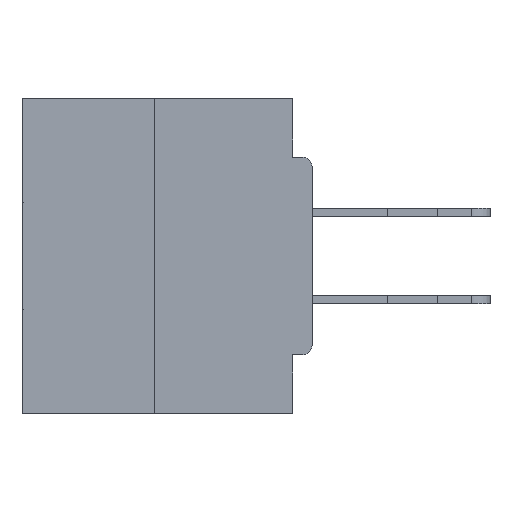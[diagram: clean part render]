
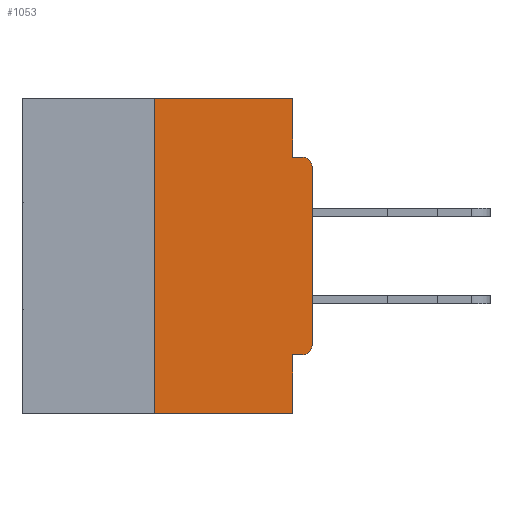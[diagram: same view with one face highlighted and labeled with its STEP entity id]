
A CAD part, left-side view. The second image highlights one B-rep face of the part: STEP entity #1053.
In plain terms, the highlighted planar face has unit normal (-1, 0, 0).
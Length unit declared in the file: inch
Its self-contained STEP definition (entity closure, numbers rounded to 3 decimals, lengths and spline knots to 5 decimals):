
#643 = VECTOR ( 'NONE', #5961, 39.37008 ) ;
#1053 = ADVANCED_FACE ( 'NONE', ( #13274 ), #39040, .F. ) ;
#1086 = EDGE_CURVE ( 'NONE', #33761, #31400, #2403, .T. ) ;
#2324 = CARTESIAN_POINT ( 'NONE',  ( 0., 0.46, 0. ) ) ;
#2388 = ORIENTED_EDGE ( 'NONE', *, *, #25637, .F. ) ;
#2403 = CIRCLE ( 'NONE', #8850, 0.015 ) ;
#2561 = DIRECTION ( 'NONE',  ( 0., 1., 0. ) ) ;
#2689 = CARTESIAN_POINT ( 'NONE',  ( 0., 0., -0.4065 ) ) ;
#2743 = EDGE_CURVE ( 'NONE', #36483, #14651, #9310, .T. ) ;
#2837 = DIRECTION ( 'NONE',  ( 0., 0., -1. ) ) ;
#3493 = LINE ( 'NONE', #24040, #643 ) ;
#4959 = VECTOR ( 'NONE', #20581, 39.37008 ) ;
#5961 = DIRECTION ( 'NONE',  ( 0., -1., 0. ) ) ;
#6221 = CARTESIAN_POINT ( 'NONE',  ( 0., 0.25, 0. ) ) ;
#6456 = LINE ( 'NONE', #2689, #19626 ) ;
#7245 = ORIENTED_EDGE ( 'NONE', *, *, #2743, .F. ) ;
#7557 = CARTESIAN_POINT ( 'NONE',  ( 0., 0.031, 0. ) ) ;
#7920 = CARTESIAN_POINT ( 'NONE',  ( 0., 0.46, -0.5 ) ) ;
#8850 = AXIS2_PLACEMENT_3D ( 'NONE', #31286, #16060, #36761 ) ;
#9133 = LINE ( 'NONE', #10523, #34714 ) ;
#9310 = LINE ( 'NONE', #14840, #13124 ) ;
#9994 = ORIENTED_EDGE ( 'NONE', *, *, #1086, .T. ) ;
#10086 = CARTESIAN_POINT ( 'NONE',  ( 0., 0., -0.3915 ) ) ;
#10115 = CARTESIAN_POINT ( 'NONE',  ( 0., 0.031, 0. ) ) ;
#10317 = DIRECTION ( 'NONE',  ( 0., 0., -1. ) ) ;
#10523 = CARTESIAN_POINT ( 'NONE',  ( 0., 0., 0. ) ) ;
#10832 = LINE ( 'NONE', #7920, #22151 ) ;
#11021 = VERTEX_POINT ( 'NONE', #20688 ) ;
#11458 = VERTEX_POINT ( 'NONE', #10115 ) ;
#11491 = LINE ( 'NONE', #6221, #30450 ) ;
#12255 = EDGE_LOOP ( 'NONE', ( #38855, #14845, #33498, #7245, #28476, #9994, #30283, #31205, #2388, #26505 ) ) ;
#13124 = VECTOR ( 'NONE', #21184, 39.37008 ) ;
#13274 = FACE_OUTER_BOUND ( 'NONE', #12255, .T. ) ;
#14538 = CARTESIAN_POINT ( 'NONE',  ( 0., 0.46, 0. ) ) ;
#14651 = VERTEX_POINT ( 'NONE', #38196 ) ;
#14840 = CARTESIAN_POINT ( 'NONE',  ( 0., 0.031, -0.5 ) ) ;
#14845 = ORIENTED_EDGE ( 'NONE', *, *, #35060, .F. ) ;
#14917 = DIRECTION ( 'NONE',  ( 1., 0., 0. ) ) ;
#15110 = DIRECTION ( 'NONE',  ( -1., 0., 0. ) ) ;
#15507 = EDGE_CURVE ( 'NONE', #11458, #36662, #22193, .T. ) ;
#15637 = EDGE_CURVE ( 'NONE', #11021, #14651, #10832, .T. ) ;
#16060 = DIRECTION ( 'NONE',  ( -1., 0., 0. ) ) ;
#16266 = CARTESIAN_POINT ( 'NONE',  ( 0., 0.031, -0.0935 ) ) ;
#16663 = AXIS2_PLACEMENT_3D ( 'NONE', #33241, #15110, #36308 ) ;
#17382 = VECTOR ( 'NONE', #10317, 39.37008 ) ;
#18173 = EDGE_CURVE ( 'NONE', #33761, #36483, #6456, .T. ) ;
#19626 = VECTOR ( 'NONE', #2561, 39.37008 ) ;
#20581 = DIRECTION ( 'NONE',  ( 0., -1., 0. ) ) ;
#20688 = CARTESIAN_POINT ( 'NONE',  ( 0., 0.25, -0.5 ) ) ;
#21145 = VERTEX_POINT ( 'NONE', #35073 ) ;
#21184 = DIRECTION ( 'NONE',  ( 0., 0., -1. ) ) ;
#22151 = VECTOR ( 'NONE', #35441, 39.37008 ) ;
#22193 = LINE ( 'NONE', #7557, #17382 ) ;
#24040 = CARTESIAN_POINT ( 'NONE',  ( 0., 0., -0.0935 ) ) ;
#24893 = VERTEX_POINT ( 'NONE', #36550 ) ;
#25481 = DIRECTION ( 'NONE',  ( 0., 0., 1. ) ) ;
#25637 = EDGE_CURVE ( 'NONE', #36662, #21145, #3493, .T. ) ;
#25737 = EDGE_CURVE ( 'NONE', #31400, #24893, #9133, .T. ) ;
#26505 = ORIENTED_EDGE ( 'NONE', *, *, #15507, .F. ) ;
#26607 = VERTEX_POINT ( 'NONE', #31741 ) ;
#28476 = ORIENTED_EDGE ( 'NONE', *, *, #18173, .F. ) ;
#29587 = CARTESIAN_POINT ( 'NONE',  ( 0., 0.015, -0.4065 ) ) ;
#30283 = ORIENTED_EDGE ( 'NONE', *, *, #25737, .T. ) ;
#30450 = VECTOR ( 'NONE', #33586, 39.37008 ) ;
#30449 = CARTESIAN_POINT ( 'NONE',  ( 0., 0.031, -0.4065 ) ) ;
#31205 = ORIENTED_EDGE ( 'NONE', *, *, #36565, .T. ) ;
#31286 = CARTESIAN_POINT ( 'NONE',  ( 0., 0.015, -0.3915 ) ) ;
#31400 = VERTEX_POINT ( 'NONE', #10086 ) ;
#31741 = CARTESIAN_POINT ( 'NONE',  ( 0., 0.25, 0. ) ) ;
#31790 = CIRCLE ( 'NONE', #16663, 0.015 ) ;
#33241 = CARTESIAN_POINT ( 'NONE',  ( 0., 0.015, -0.1085 ) ) ;
#33498 = ORIENTED_EDGE ( 'NONE', *, *, #15637, .T. ) ;
#33586 = DIRECTION ( 'NONE',  ( 0., 0., 1. ) ) ;
#33729 = AXIS2_PLACEMENT_3D ( 'NONE', #14538, #14917, #2837 ) ;
#33761 = VERTEX_POINT ( 'NONE', #29587 ) ;
#33829 = LINE ( 'NONE', #2324, #4959 ) ;
#34714 = VECTOR ( 'NONE', #25481, 39.37008 ) ;
#35060 = EDGE_CURVE ( 'NONE', #11021, #26607, #11491, .T. ) ;
#35073 = CARTESIAN_POINT ( 'NONE',  ( 0., 0.015, -0.0935 ) ) ;
#35441 = DIRECTION ( 'NONE',  ( 0., -1., 0. ) ) ;
#36308 = DIRECTION ( 'NONE',  ( 0., 0., -1. ) ) ;
#36483 = VERTEX_POINT ( 'NONE', #30449 ) ;
#36550 = CARTESIAN_POINT ( 'NONE',  ( 0., 0., -0.1085 ) ) ;
#36565 = EDGE_CURVE ( 'NONE', #24893, #21145, #31790, .T. ) ;
#36662 = VERTEX_POINT ( 'NONE', #16266 ) ;
#36761 = DIRECTION ( 'NONE',  ( 0., 0., -1. ) ) ;
#36813 = EDGE_CURVE ( 'NONE', #26607, #11458, #33829, .T. ) ;
#38196 = CARTESIAN_POINT ( 'NONE',  ( 0., 0.031, -0.5 ) ) ;
#38855 = ORIENTED_EDGE ( 'NONE', *, *, #36813, .F. ) ;
#39040 = PLANE ( 'NONE',  #33729 ) ;
